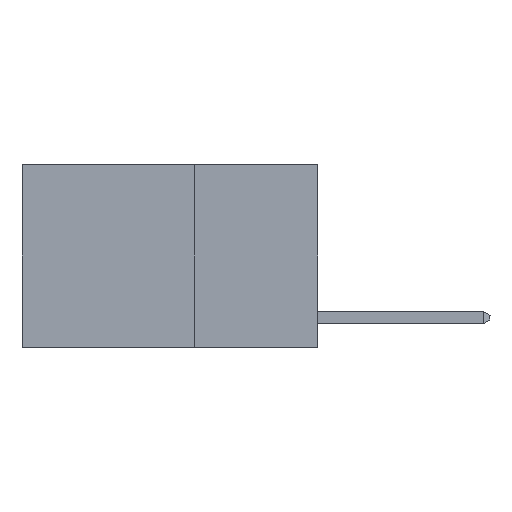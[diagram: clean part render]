
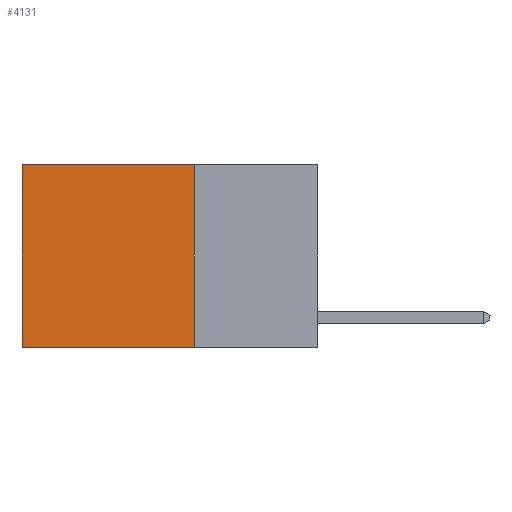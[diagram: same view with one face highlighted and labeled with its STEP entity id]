
A CAD part, left-side view. The second image highlights one B-rep face of the part: STEP entity #4131.
In plain terms, the highlighted planar face has unit normal (-1, 0, 0).
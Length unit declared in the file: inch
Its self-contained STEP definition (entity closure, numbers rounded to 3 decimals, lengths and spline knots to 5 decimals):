
#120 = DIRECTION ( 'NONE',  ( 0., 0., -1. ) ) ;
#1889 = VERTEX_POINT ( 'NONE', #10891 ) ;
#2314 = EDGE_CURVE ( 'NONE', #1889, #23774, #9313, .T. ) ;
#2427 = LINE ( 'NONE', #18236, #25513 ) ;
#2569 = DIRECTION ( 'NONE',  ( 0., 1., 0. ) ) ;
#2617 = VECTOR ( 'NONE', #120, 39.37008 ) ;
#2944 = AXIS2_PLACEMENT_3D ( 'NONE', #15563, #18108, #27179 ) ;
#3428 = CARTESIAN_POINT ( 'NONE',  ( 0.2625, 0.6, -0.37 ) ) ;
#3852 = CARTESIAN_POINT ( 'NONE',  ( 0.2625, 0.6, 0. ) ) ;
#4131 = ADVANCED_FACE ( 'NONE', ( #8977 ), #11072, .F. ) ;
#6743 = VERTEX_POINT ( 'NONE', #8867 ) ;
#6811 = CARTESIAN_POINT ( 'NONE',  ( 0.2625, 0.25, -0.37 ) ) ;
#8867 = CARTESIAN_POINT ( 'NONE',  ( 0.2625, 0.6, 0. ) ) ;
#8977 = FACE_OUTER_BOUND ( 'NONE', #20914, .T. ) ;
#8996 = LINE ( 'NONE', #20349, #24738 ) ;
#9313 = LINE ( 'NONE', #21910, #2617 ) ;
#10380 = LINE ( 'NONE', #3852, #22266 ) ;
#10891 = CARTESIAN_POINT ( 'NONE',  ( 0.2625, 0.25, 0. ) ) ;
#11072 = PLANE ( 'NONE',  #2944 ) ;
#14815 = ORIENTED_EDGE ( 'NONE', *, *, #2314, .F. ) ;
#15563 = CARTESIAN_POINT ( 'NONE',  ( 0.2625, 0.25, 0. ) ) ;
#15895 = VERTEX_POINT ( 'NONE', #3428 ) ;
#16529 = EDGE_CURVE ( 'NONE', #23774, #15895, #8996, .T. ) ;
#18108 = DIRECTION ( 'NONE',  ( 1., 0., 0. ) ) ;
#18236 = CARTESIAN_POINT ( 'NONE',  ( 0.2625, 0.25, 0. ) ) ;
#19376 = ORIENTED_EDGE ( 'NONE', *, *, #16529, .F. ) ;
#20349 = CARTESIAN_POINT ( 'NONE',  ( 0.2625, 0.25, -0.37 ) ) ;
#20914 = EDGE_LOOP ( 'NONE', ( #26692, #19376, #14815, #25446 ) ) ;
#21910 = CARTESIAN_POINT ( 'NONE',  ( 0.2625, 0.25, 0. ) ) ;
#22018 = DIRECTION ( 'NONE',  ( 0., 0., -1. ) ) ;
#22266 = VECTOR ( 'NONE', #22018, 39.37008 ) ;
#23774 = VERTEX_POINT ( 'NONE', #6811 ) ;
#24738 = VECTOR ( 'NONE', #26745, 39.37008 ) ;
#25446 = ORIENTED_EDGE ( 'NONE', *, *, #26689, .T. ) ;
#25513 = VECTOR ( 'NONE', #2569, 39.37008 ) ;
#26689 = EDGE_CURVE ( 'NONE', #1889, #6743, #2427, .T. ) ;
#26692 = ORIENTED_EDGE ( 'NONE', *, *, #28660, .T. ) ;
#26745 = DIRECTION ( 'NONE',  ( 0., 1., 0. ) ) ;
#27179 = DIRECTION ( 'NONE',  ( 0., 0., -1. ) ) ;
#28660 = EDGE_CURVE ( 'NONE', #6743, #15895, #10380, .T. ) ;
